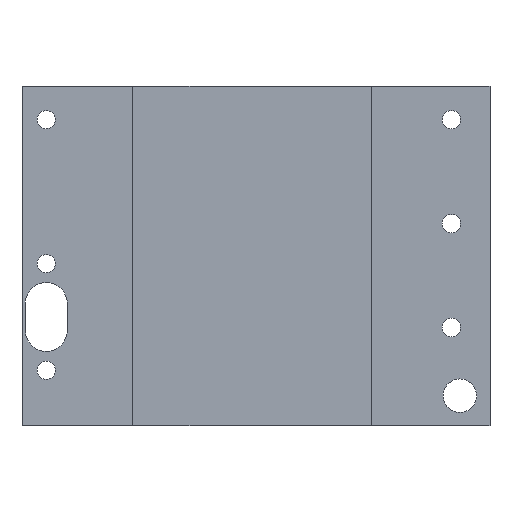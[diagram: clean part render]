
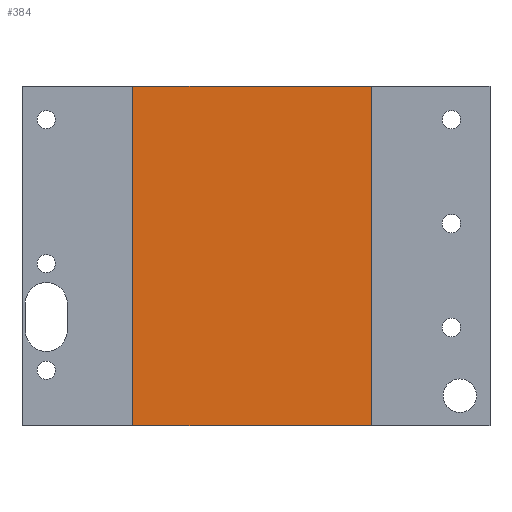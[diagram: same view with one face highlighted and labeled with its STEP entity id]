
A CAD part, front view. The second image highlights one B-rep face of the part: STEP entity #384.
In plain terms, the highlighted planar face has unit normal (0, -1, 0).
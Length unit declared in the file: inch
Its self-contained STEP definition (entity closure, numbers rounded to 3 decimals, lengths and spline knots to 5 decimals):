
#39 = CARTESIAN_POINT ( 'NONE',  ( 2.605, 0.018, 0. ) ) ;
#57 = EDGE_CURVE ( 'NONE', #300, #130, #995, .T. ) ;
#130 = VERTEX_POINT ( 'NONE', #782 ) ;
#143 = DIRECTION ( 'NONE',  ( 0., 1., 0. ) ) ;
#204 = ORIENTED_EDGE ( 'NONE', *, *, #702, .F. ) ;
#225 = AXIS2_PLACEMENT_3D ( 'NONE', #938, #143, #940 ) ;
#273 = EDGE_CURVE ( 'NONE', #526, #595, #929, .T. ) ;
#282 = ORIENTED_EDGE ( 'NONE', *, *, #273, .T. ) ;
#300 = VERTEX_POINT ( 'NONE', #923 ) ;
#374 = EDGE_LOOP ( 'NONE', ( #282, #204, #447, #602 ) ) ;
#384 = ADVANCED_FACE ( 'NONE', ( #874 ), #942, .F. ) ;
#447 = ORIENTED_EDGE ( 'NONE', *, *, #57, .F. ) ;
#459 = DIRECTION ( 'NONE',  ( 1., 0., 0. ) ) ;
#481 = VECTOR ( 'NONE', #459, 39.37008 ) ;
#484 = LINE ( 'NONE', #495, #481 ) ;
#487 = CARTESIAN_POINT ( 'NONE',  ( 0.827, 0.018, 0. ) ) ;
#495 = CARTESIAN_POINT ( 'NONE',  ( 0., 0.018, -2.534 ) ) ;
#498 = VECTOR ( 'NONE', #531, 39.37008 ) ;
#520 = CARTESIAN_POINT ( 'NONE',  ( 0., 0.018, 0. ) ) ;
#524 = LINE ( 'NONE', #520, #498 ) ;
#526 = VERTEX_POINT ( 'NONE', #825 ) ;
#531 = DIRECTION ( 'NONE',  ( 1., 0., 0. ) ) ;
#533 = DIRECTION ( 'NONE',  ( 0., 0., 1. ) ) ;
#595 = VERTEX_POINT ( 'NONE', #39 ) ;
#602 = ORIENTED_EDGE ( 'NONE', *, *, #714, .T. ) ;
#702 = EDGE_CURVE ( 'NONE', #130, #595, #524, .T. ) ;
#714 = EDGE_CURVE ( 'NONE', #300, #526, #484, .T. ) ;
#782 = CARTESIAN_POINT ( 'NONE',  ( 0.827, 0.018, 0. ) ) ;
#825 = CARTESIAN_POINT ( 'NONE',  ( 2.605, 0.018, -2.534 ) ) ;
#874 = FACE_OUTER_BOUND ( 'NONE', #374, .T. ) ;
#923 = CARTESIAN_POINT ( 'NONE',  ( 0.827, 0.018, -2.534 ) ) ;
#926 = CARTESIAN_POINT ( 'NONE',  ( 2.605, 0.018, 0. ) ) ;
#929 = LINE ( 'NONE', #926, #974 ) ;
#932 = DIRECTION ( 'NONE',  ( 0., 0., 1. ) ) ;
#938 = CARTESIAN_POINT ( 'NONE',  ( 0., 0.018, 0. ) ) ;
#940 = DIRECTION ( 'NONE',  ( 0., 0., 1. ) ) ;
#942 = PLANE ( 'NONE',  #225 ) ;
#974 = VECTOR ( 'NONE', #932, 39.37008 ) ;
#989 = VECTOR ( 'NONE', #533, 39.37008 ) ;
#995 = LINE ( 'NONE', #487, #989 ) ;
